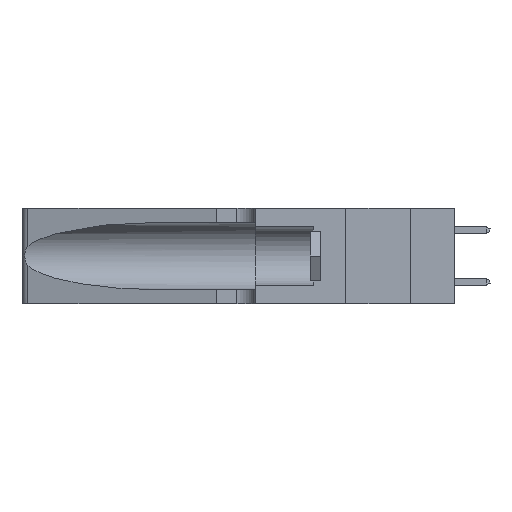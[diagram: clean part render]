
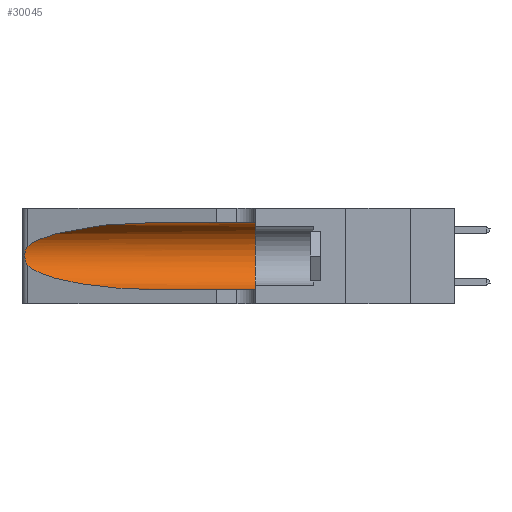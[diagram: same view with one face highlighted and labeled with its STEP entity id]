
A CAD part, left-side view. The second image highlights one B-rep face of the part: STEP entity #30045.
In plain terms, the highlighted cylindrical face has radius 3.308 mm (diameter 6.617 mm), a partial arc.
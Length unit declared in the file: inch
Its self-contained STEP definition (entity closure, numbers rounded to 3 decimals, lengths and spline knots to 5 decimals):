
#145 = CARTESIAN_POINT ( 'NONE',  ( 0.1305, 1.61858, 0.31525 ) ) ;
#207 = AXIS2_PLACEMENT_3D ( 'NONE', #19778, #4921, #22275 ) ;
#227 = CARTESIAN_POINT ( 'NONE',  ( 0.18966, 0.96281, 0.05475 ) ) ;
#399 = EDGE_CURVE ( 'NONE', #5460, #21320, #27948, .T. ) ;
#1119 = CARTESIAN_POINT ( 'NONE',  ( 0.18966, 0.96281, 0.31525 ) ) ;
#1791 = CARTESIAN_POINT ( 'NONE',  ( 0.26018, 1.23835, 0.19895 ) ) ;
#4320 = CARTESIAN_POINT ( 'NONE',  ( 0.26075, 1.23896, 0.178 ) ) ;
#4921 = DIRECTION ( 'NONE',  ( 0., 1., 0. ) ) ;
#5460 = VERTEX_POINT ( 'NONE', #27727 ) ;
#6163 = CARTESIAN_POINT ( 'NONE',  ( 0.25487, 1.22718, 0.22369 ) ) ;
#6817 = CARTESIAN_POINT ( 'NONE',  ( 0.25856, 1.23593, 0.16098 ) ) ;
#7080 = EDGE_CURVE ( 'NONE', #25021, #22865, #13082, .T. ) ;
#8063 = CARTESIAN_POINT ( 'NONE',  ( 0.1305, 0.72297, 0.05475 ) ) ;
#8391 =( BOUNDED_CURVE ( )  B_SPLINE_CURVE ( 3, ( #12718, #27443, #227, #17678 ),
 .UNSPECIFIED., .F., .F. ) 
 B_SPLINE_CURVE_WITH_KNOTS ( ( 4, 4 ),
 ( 3.44316, 4.71239 ),
 .UNSPECIFIED. ) 
 CURVE ( )  GEOMETRIC_REPRESENTATION_ITEM ( )  RATIONAL_B_SPLINE_CURVE ( ( 1., 0.87, 0.87, 1. ) ) 
 REPRESENTATION_ITEM ( '' )  );
#8591 = VECTOR ( 'NONE', #8774, 39.37008 ) ;
#8774 = DIRECTION ( 'NONE',  ( 0., -1., 0. ) ) ;
#9205 = CARTESIAN_POINT ( 'NONE',  ( 0.25487, 1.22718, 0.22369 ) ) ;
#9315 = CARTESIAN_POINT ( 'NONE',  ( 0.25639, 1.23186, 0.15144 ) ) ;
#11067 = CARTESIAN_POINT ( 'NONE',  ( 0.1305, 0.72297, 0.31525 ) ) ;
#11838 = CARTESIAN_POINT ( 'NONE',  ( 0.25487, 1.22718, 0.14631 ) ) ;
#12403 = EDGE_LOOP ( 'NONE', ( #30084, #16700, #14794, #23628, #16094, #15210 ) ) ;
#12718 = CARTESIAN_POINT ( 'NONE',  ( 0.25487, 1.22718, 0.14631 ) ) ;
#13082 = CIRCLE ( 'NONE', #207, 0.13025 ) ;
#13929 = LINE ( 'NONE', #145, #25444 ) ;
#14057 = CARTESIAN_POINT ( 'NONE',  ( 0.25487, 1.22718, 0.14631 ) ) ;
#14232 = CARTESIAN_POINT ( 'NONE',  ( 0.25639, 1.23184, 0.21858 ) ) ;
#14307 = EDGE_CURVE ( 'NONE', #21320, #24670, #8391, .T. ) ;
#14794 = ORIENTED_EDGE ( 'NONE', *, *, #14307, .T. ) ;
#15210 = ORIENTED_EDGE ( 'NONE', *, *, #23568, .F. ) ;
#16094 = ORIENTED_EDGE ( 'NONE', *, *, #7080, .F. ) ;
#16501 = VERTEX_POINT ( 'NONE', #30014 ) ;
#16700 = ORIENTED_EDGE ( 'NONE', *, *, #399, .T. ) ;
#16704 = CARTESIAN_POINT ( 'NONE',  ( 0.25854, 1.2359, 0.20912 ) ) ;
#17616 = DIRECTION ( 'NONE',  ( 0., -1., 0. ) ) ;
#17678 = CARTESIAN_POINT ( 'NONE',  ( 0.1305, 0.72297, 0.05475 ) ) ;
#17770 = CYLINDRICAL_SURFACE ( 'NONE', #27558, 0.13025 ) ;
#19175 = CARTESIAN_POINT ( 'NONE',  ( 0.26075, 1.23896, 0.19203 ) ) ;
#19778 = CARTESIAN_POINT ( 'NONE',  ( 0.1305, 0.35, 0.185 ) ) ;
#19799 = DIRECTION ( 'NONE',  ( 0., 0., -1. ) ) ;
#21009 = CARTESIAN_POINT ( 'NONE',  ( 0.2373, 1.15595, 0.28018 ) ) ;
#21320 = VERTEX_POINT ( 'NONE', #14057 ) ;
#21673 = CARTESIAN_POINT ( 'NONE',  ( 0.26017, 1.23833, 0.17102 ) ) ;
#22275 = DIRECTION ( 'NONE',  ( 0., 0., 1. ) ) ;
#22422 = CARTESIAN_POINT ( 'NONE',  ( 0.1305, 0.35, 0.05475 ) ) ;
#22464 = EDGE_CURVE ( 'NONE', #16501, #5460, #28923, .T. ) ;
#22865 = VERTEX_POINT ( 'NONE', #22422 ) ;
#23568 = EDGE_CURVE ( 'NONE', #16501, #25021, #13929, .T. ) ;
#23628 = ORIENTED_EDGE ( 'NONE', *, *, #27460, .T. ) ;
#24112 = CARTESIAN_POINT ( 'NONE',  ( 0.25789, 1.23486, 0.15765 ) ) ;
#24670 = VERTEX_POINT ( 'NONE', #8063 ) ;
#24709 = DIRECTION ( 'NONE',  ( 0., -1., 0. ) ) ;
#25021 = VERTEX_POINT ( 'NONE', #29044 ) ;
#25063 = FACE_OUTER_BOUND ( 'NONE', #12403, .T. ) ;
#25444 = VECTOR ( 'NONE', #17616, 39.37008 ) ;
#26024 = CARTESIAN_POINT ( 'NONE',  ( 0.1305, 1.61858, 0.05475 ) ) ;
#26569 = CARTESIAN_POINT ( 'NONE',  ( 0.25555, 1.22993, 0.14849 ) ) ;
#27175 = CARTESIAN_POINT ( 'NONE',  ( 0.1305, 1.61858, 0.185 ) ) ;
#27443 = CARTESIAN_POINT ( 'NONE',  ( 0.2373, 1.15595, 0.08982 ) ) ;
#27460 = EDGE_CURVE ( 'NONE', #24670, #22865, #28252, .T. ) ;
#27558 = AXIS2_PLACEMENT_3D ( 'NONE', #27175, #24709, #19799 ) ;
#27727 = CARTESIAN_POINT ( 'NONE',  ( 0.25487, 1.22718, 0.22369 ) ) ;
#27948 = B_SPLINE_CURVE_WITH_KNOTS ( 'NONE', 3,
 ( #9205, #28901, #14232, #31367, #16704, #1791, #19175, #4320, #21673, #6817, #24112, #9315, #26569, #11838 ),
 .UNSPECIFIED., .F., .F.,
 ( 4, 2, 2, 2, 2, 2, 4 ),
 ( 0., 0.00027, 0.00053, 0.00107, 0.0016, 0.00187, 0.00214 ),
 .UNSPECIFIED. ) ;
#28252 = LINE ( 'NONE', #26024, #8591 ) ;
#28901 = CARTESIAN_POINT ( 'NONE',  ( 0.25555, 1.22994, 0.2215 ) ) ;
#28923 =( BOUNDED_CURVE ( )  B_SPLINE_CURVE ( 3, ( #11067, #1119, #21009, #6163 ),
 .UNSPECIFIED., .F., .F. ) 
 B_SPLINE_CURVE_WITH_KNOTS ( ( 4, 4 ),
 ( 1.5708, 2.84003 ),
 .UNSPECIFIED. ) 
 CURVE ( )  GEOMETRIC_REPRESENTATION_ITEM ( )  RATIONAL_B_SPLINE_CURVE ( ( 1., 0.87, 0.87, 1. ) ) 
 REPRESENTATION_ITEM ( '' )  );
#29044 = CARTESIAN_POINT ( 'NONE',  ( 0.1305, 0.35, 0.31525 ) ) ;
#30014 = CARTESIAN_POINT ( 'NONE',  ( 0.1305, 0.72297, 0.31525 ) ) ;
#30045 = ADVANCED_FACE ( 'NONE', ( #25063 ), #17770, .F. ) ;
#30084 = ORIENTED_EDGE ( 'NONE', *, *, #22464, .T. ) ;
#31367 = CARTESIAN_POINT ( 'NONE',  ( 0.25787, 1.23484, 0.2124 ) ) ;
